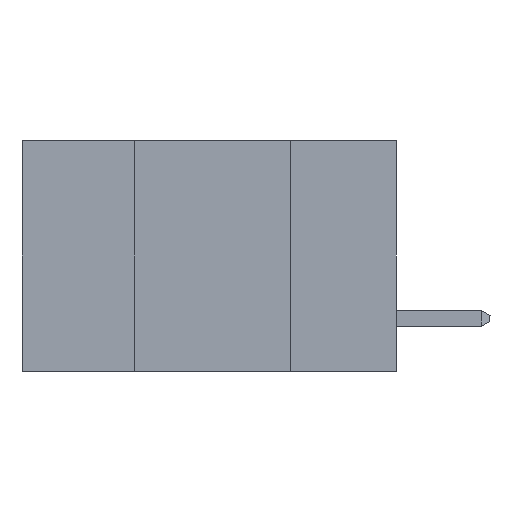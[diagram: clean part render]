
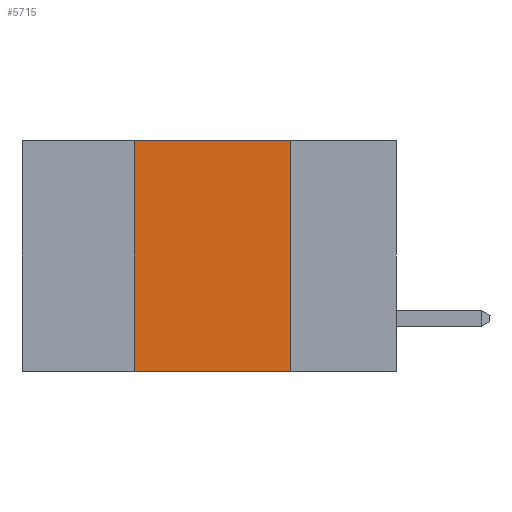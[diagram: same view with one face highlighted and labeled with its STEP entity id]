
A CAD part, left-side view. The second image highlights one B-rep face of the part: STEP entity #5715.
In plain terms, the highlighted planar face has unit normal (-1, 0, 0).
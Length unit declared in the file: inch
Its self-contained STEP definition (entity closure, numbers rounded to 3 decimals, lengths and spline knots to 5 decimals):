
#432 = DIRECTION ( 'NONE',  ( 0., 0., 1. ) ) ;
#510 = LINE ( 'NONE', #11319, #8649 ) ;
#710 = VERTEX_POINT ( 'NONE', #2241 ) ;
#713 = ORIENTED_EDGE ( 'NONE', *, *, #3818, .F. ) ;
#1037 = ORIENTED_EDGE ( 'NONE', *, *, #14841, .T. ) ;
#1670 = AXIS2_PLACEMENT_3D ( 'NONE', #12780, #6748, #11590 ) ;
#2241 = CARTESIAN_POINT ( 'NONE',  ( 0., 0.17, -0.37 ) ) ;
#2392 = ORIENTED_EDGE ( 'NONE', *, *, #14695, .F. ) ;
#2886 = VECTOR ( 'NONE', #4280, 39.37008 ) ;
#3130 = VERTEX_POINT ( 'NONE', #11748 ) ;
#3818 = EDGE_CURVE ( 'NONE', #6944, #710, #6925, .T. ) ;
#4280 = DIRECTION ( 'NONE',  ( 0., 0., -1. ) ) ;
#5715 = ADVANCED_FACE ( 'NONE', ( #7949 ), #9212, .F. ) ;
#6748 = DIRECTION ( 'NONE',  ( 1., 0., 0. ) ) ;
#6844 = VERTEX_POINT ( 'NONE', #11196 ) ;
#6880 = DIRECTION ( 'NONE',  ( 0., -1., 0. ) ) ;
#6886 = ORIENTED_EDGE ( 'NONE', *, *, #11772, .F. ) ;
#6925 = LINE ( 'NONE', #14151, #2886 ) ;
#6944 = VERTEX_POINT ( 'NONE', #14057 ) ;
#7903 = VECTOR ( 'NONE', #6880, 39.37008 ) ;
#7949 = FACE_OUTER_BOUND ( 'NONE', #10136, .T. ) ;
#8084 = LINE ( 'NONE', #15141, #7903 ) ;
#8649 = VECTOR ( 'NONE', #432, 39.37008 ) ;
#9212 = PLANE ( 'NONE',  #1670 ) ;
#10136 = EDGE_LOOP ( 'NONE', ( #713, #6886, #2392, #1037 ) ) ;
#10226 = LINE ( 'NONE', #11573, #14512 ) ;
#11196 = CARTESIAN_POINT ( 'NONE',  ( 0., 0.42, -0.37 ) ) ;
#11319 = CARTESIAN_POINT ( 'NONE',  ( 0., 0.42, -0.37 ) ) ;
#11573 = CARTESIAN_POINT ( 'NONE',  ( 0., 0.6, 0. ) ) ;
#11590 = DIRECTION ( 'NONE',  ( 0., 0., -1. ) ) ;
#11748 = CARTESIAN_POINT ( 'NONE',  ( 0., 0.42, 0. ) ) ;
#11772 = EDGE_CURVE ( 'NONE', #3130, #6944, #10226, .T. ) ;
#12598 = DIRECTION ( 'NONE',  ( 0., -1., 0. ) ) ;
#12780 = CARTESIAN_POINT ( 'NONE',  ( 0., 0.6, 0. ) ) ;
#14057 = CARTESIAN_POINT ( 'NONE',  ( 0., 0.17, 0. ) ) ;
#14151 = CARTESIAN_POINT ( 'NONE',  ( 0., 0.17, -0.37 ) ) ;
#14512 = VECTOR ( 'NONE', #12598, 39.37008 ) ;
#14695 = EDGE_CURVE ( 'NONE', #6844, #3130, #510, .T. ) ;
#14841 = EDGE_CURVE ( 'NONE', #6844, #710, #8084, .T. ) ;
#15141 = CARTESIAN_POINT ( 'NONE',  ( 0., 0.6, -0.37 ) ) ;
